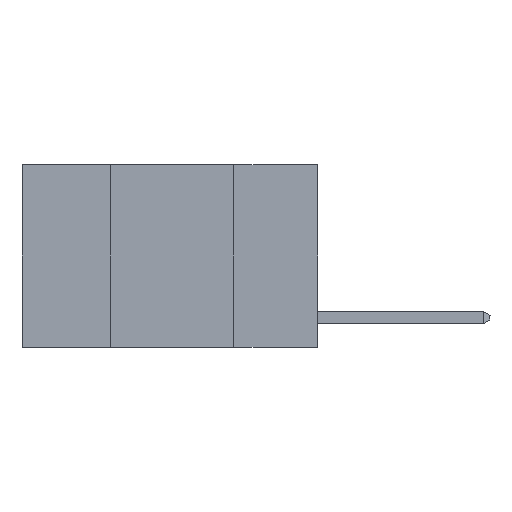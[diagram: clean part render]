
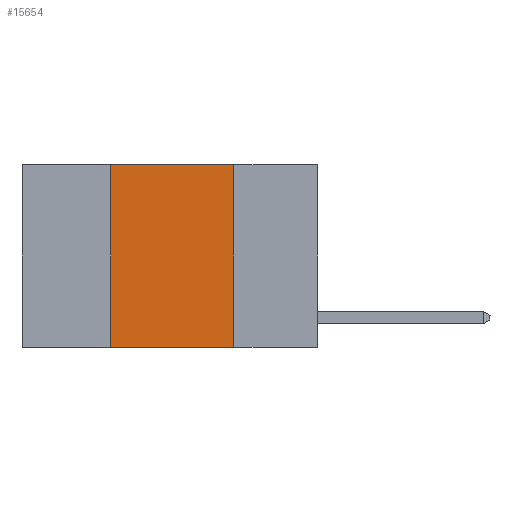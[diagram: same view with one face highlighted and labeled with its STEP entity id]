
A CAD part, left-side view. The second image highlights one B-rep face of the part: STEP entity #15654.
In plain terms, the highlighted planar face has unit normal (-1, 0, 0).
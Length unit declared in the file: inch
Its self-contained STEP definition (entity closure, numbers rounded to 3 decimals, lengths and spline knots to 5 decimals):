
#25 = AXIS2_PLACEMENT_3D ( 'NONE', #29053, #2267, #9048 ) ;
#265 = EDGE_CURVE ( 'NONE', #11594, #5195, #19093, .T. ) ;
#1548 = EDGE_LOOP ( 'NONE', ( #7127, #10837, #2092, #28513 ) ) ;
#2092 = ORIENTED_EDGE ( 'NONE', *, *, #8254, .F. ) ;
#2267 = DIRECTION ( 'NONE',  ( 1., 0., 0. ) ) ;
#2463 = CARTESIAN_POINT ( 'NONE',  ( 0., 0.42, 0. ) ) ;
#2606 = LINE ( 'NONE', #22616, #14821 ) ;
#2739 = LINE ( 'NONE', #25248, #28677 ) ;
#5195 = VERTEX_POINT ( 'NONE', #5399 ) ;
#5399 = CARTESIAN_POINT ( 'NONE',  ( 0., 0.17, -0.37 ) ) ;
#6313 = CARTESIAN_POINT ( 'NONE',  ( 0., 0.17, 0. ) ) ;
#6759 = CARTESIAN_POINT ( 'NONE',  ( 0., 0.42, 0. ) ) ;
#6965 = VERTEX_POINT ( 'NONE', #18880 ) ;
#7127 = ORIENTED_EDGE ( 'NONE', *, *, #265, .F. ) ;
#8254 = EDGE_CURVE ( 'NONE', #6965, #14953, #27473, .T. ) ;
#9048 = DIRECTION ( 'NONE',  ( 0., 0., -1. ) ) ;
#10837 = ORIENTED_EDGE ( 'NONE', *, *, #21843, .F. ) ;
#11594 = VERTEX_POINT ( 'NONE', #6313 ) ;
#11724 = DIRECTION ( 'NONE',  ( 0., -1., 0. ) ) ;
#12488 = DIRECTION ( 'NONE',  ( 0., 0., -1. ) ) ;
#13642 = DIRECTION ( 'NONE',  ( 0., -1., 0. ) ) ;
#14821 = VECTOR ( 'NONE', #13642, 39.37008 ) ;
#14953 = VERTEX_POINT ( 'NONE', #6759 ) ;
#15251 = EDGE_CURVE ( 'NONE', #6965, #5195, #2739, .T. ) ;
#15536 = FACE_OUTER_BOUND ( 'NONE', #1548, .T. ) ;
#15654 = ADVANCED_FACE ( 'NONE', ( #15536 ), #22860, .F. ) ;
#18880 = CARTESIAN_POINT ( 'NONE',  ( 0., 0.42, -0.37 ) ) ;
#19093 = LINE ( 'NONE', #25877, #24725 ) ;
#20241 = VECTOR ( 'NONE', #20261, 39.37008 ) ;
#20261 = DIRECTION ( 'NONE',  ( 0., 0., 1. ) ) ;
#21843 = EDGE_CURVE ( 'NONE', #14953, #11594, #2606, .T. ) ;
#22616 = CARTESIAN_POINT ( 'NONE',  ( 0., 0.6, 0. ) ) ;
#22860 = PLANE ( 'NONE',  #25 ) ;
#24725 = VECTOR ( 'NONE', #12488, 39.37008 ) ;
#25248 = CARTESIAN_POINT ( 'NONE',  ( 0., 0.6, -0.37 ) ) ;
#25877 = CARTESIAN_POINT ( 'NONE',  ( 0., 0.17, 0. ) ) ;
#27473 = LINE ( 'NONE', #2463, #20241 ) ;
#28513 = ORIENTED_EDGE ( 'NONE', *, *, #15251, .T. ) ;
#28677 = VECTOR ( 'NONE', #11724, 39.37008 ) ;
#29053 = CARTESIAN_POINT ( 'NONE',  ( 0., 0.6, 0. ) ) ;
